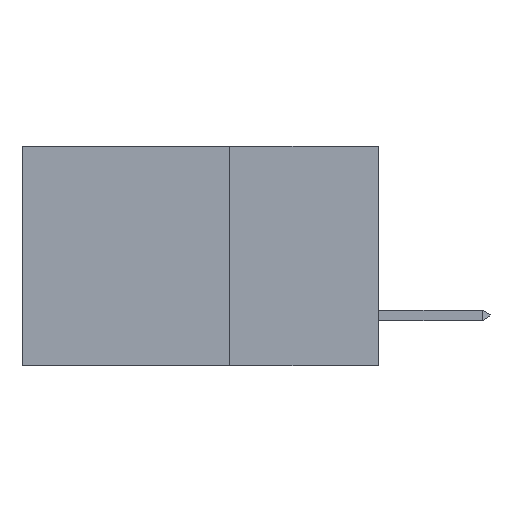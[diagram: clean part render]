
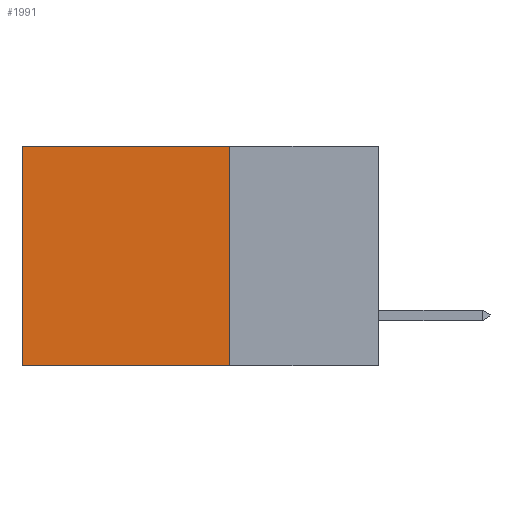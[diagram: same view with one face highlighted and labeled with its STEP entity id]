
A CAD part, left-side view. The second image highlights one B-rep face of the part: STEP entity #1991.
In plain terms, the highlighted planar face has unit normal (-1, 0, 0).
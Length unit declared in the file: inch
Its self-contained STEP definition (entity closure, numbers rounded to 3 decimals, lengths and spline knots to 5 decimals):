
#149 = VECTOR ( 'NONE', #7773, 39.37008 ) ;
#332 = ORIENTED_EDGE ( 'NONE', *, *, #13582, .F. ) ;
#507 = LINE ( 'NONE', #3129, #3149 ) ;
#1148 = CARTESIAN_POINT ( 'NONE',  ( 0.298, 0.25, 0. ) ) ;
#1646 = CARTESIAN_POINT ( 'NONE',  ( 0.298, 0.25, 0. ) ) ;
#1731 = LINE ( 'NONE', #1148, #149 ) ;
#1991 = ADVANCED_FACE ( 'NONE', ( #10430 ), #6790, .F. ) ;
#3129 = CARTESIAN_POINT ( 'NONE',  ( 0.298, 0.25, 0. ) ) ;
#3149 = VECTOR ( 'NONE', #5398, 39.37008 ) ;
#3445 = AXIS2_PLACEMENT_3D ( 'NONE', #1646, #11910, #13039 ) ;
#3699 = CARTESIAN_POINT ( 'NONE',  ( 0.298, 0.6, -0.37 ) ) ;
#4175 = LINE ( 'NONE', #12621, #4522 ) ;
#4469 = ORIENTED_EDGE ( 'NONE', *, *, #9825, .T. ) ;
#4522 = VECTOR ( 'NONE', #6960, 39.37008 ) ;
#5398 = DIRECTION ( 'NONE',  ( 0., 0., -1. ) ) ;
#5711 = EDGE_CURVE ( 'NONE', #12822, #11845, #11388, .T. ) ;
#6790 = PLANE ( 'NONE',  #3445 ) ;
#6960 = DIRECTION ( 'NONE',  ( 0., 0., -1. ) ) ;
#7326 = ORIENTED_EDGE ( 'NONE', *, *, #14179, .T. ) ;
#7773 = DIRECTION ( 'NONE',  ( 0., 1., 0. ) ) ;
#8290 = ORIENTED_EDGE ( 'NONE', *, *, #5711, .F. ) ;
#9593 = VERTEX_POINT ( 'NONE', #10608 ) ;
#9818 = VECTOR ( 'NONE', #10637, 39.37008 ) ;
#9825 = EDGE_CURVE ( 'NONE', #12504, #9593, #1731, .T. ) ;
#10430 = FACE_OUTER_BOUND ( 'NONE', #11131, .T. ) ;
#10608 = CARTESIAN_POINT ( 'NONE',  ( 0.298, 0.6, 0. ) ) ;
#10637 = DIRECTION ( 'NONE',  ( 0., 1., 0. ) ) ;
#11131 = EDGE_LOOP ( 'NONE', ( #7326, #8290, #332, #4469 ) ) ;
#11249 = CARTESIAN_POINT ( 'NONE',  ( 0.298, 0.25, -0.37 ) ) ;
#11388 = LINE ( 'NONE', #14064, #9818 ) ;
#11845 = VERTEX_POINT ( 'NONE', #3699 ) ;
#11910 = DIRECTION ( 'NONE',  ( 1., 0., 0. ) ) ;
#12504 = VERTEX_POINT ( 'NONE', #14188 ) ;
#12621 = CARTESIAN_POINT ( 'NONE',  ( 0.298, 0.6, 0. ) ) ;
#12822 = VERTEX_POINT ( 'NONE', #11249 ) ;
#13039 = DIRECTION ( 'NONE',  ( 0., 0., -1. ) ) ;
#13582 = EDGE_CURVE ( 'NONE', #12504, #12822, #507, .T. ) ;
#14064 = CARTESIAN_POINT ( 'NONE',  ( 0.298, 0.25, -0.37 ) ) ;
#14179 = EDGE_CURVE ( 'NONE', #9593, #11845, #4175, .T. ) ;
#14188 = CARTESIAN_POINT ( 'NONE',  ( 0.298, 0.25, 0. ) ) ;
